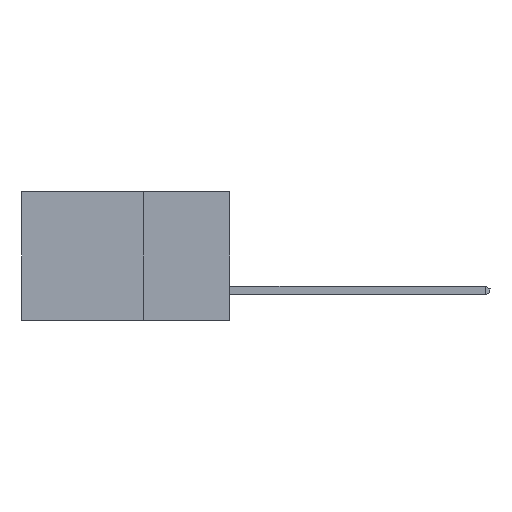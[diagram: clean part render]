
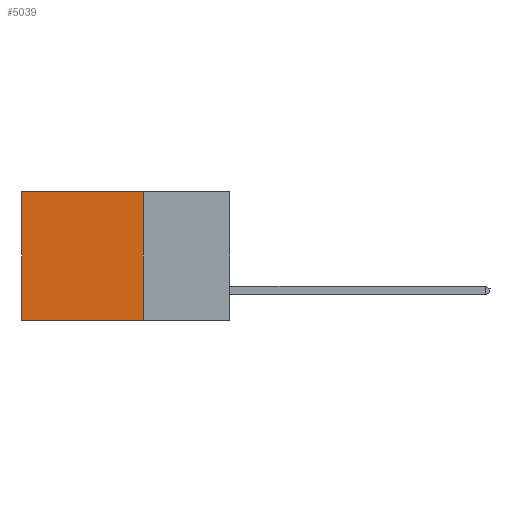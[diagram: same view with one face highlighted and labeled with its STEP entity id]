
A CAD part, left-side view. The second image highlights one B-rep face of the part: STEP entity #5039.
In plain terms, the highlighted planar face has unit normal (-1, 0, 0).
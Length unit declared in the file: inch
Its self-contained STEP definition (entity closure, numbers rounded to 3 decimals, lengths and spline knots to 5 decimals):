
#71 = AXIS2_PLACEMENT_3D ( 'NONE', #5232, #5134, #6572 ) ;
#992 = CARTESIAN_POINT ( 'NONE',  ( 0.298, 0.25, 0. ) ) ;
#1213 = CARTESIAN_POINT ( 'NONE',  ( 0.298, 0.6, -0.37 ) ) ;
#1658 = EDGE_CURVE ( 'NONE', #10944, #4196, #7610, .T. ) ;
#3226 = VECTOR ( 'NONE', #11026, 39.37008 ) ;
#4196 = VERTEX_POINT ( 'NONE', #11850 ) ;
#4516 = CARTESIAN_POINT ( 'NONE',  ( 0.298, 0.6, 0. ) ) ;
#4871 = DIRECTION ( 'NONE',  ( 0., 1., 0. ) ) ;
#5039 = ADVANCED_FACE ( 'NONE', ( #14715 ), #13053, .F. ) ;
#5134 = DIRECTION ( 'NONE',  ( 1., 0., 0. ) ) ;
#5232 = CARTESIAN_POINT ( 'NONE',  ( 0.298, 0.25, 0. ) ) ;
#6140 = EDGE_CURVE ( 'NONE', #4196, #11334, #9759, .T. ) ;
#6254 = EDGE_CURVE ( 'NONE', #7021, #11334, #13254, .T. ) ;
#6343 = DIRECTION ( 'NONE',  ( 0., 0., -1. ) ) ;
#6572 = DIRECTION ( 'NONE',  ( 0., 0., -1. ) ) ;
#7021 = VERTEX_POINT ( 'NONE', #11806 ) ;
#7163 = CARTESIAN_POINT ( 'NONE',  ( 0.298, 0.25, -0.37 ) ) ;
#7186 = VECTOR ( 'NONE', #4871, 39.37008 ) ;
#7610 = LINE ( 'NONE', #992, #15599 ) ;
#7684 = CARTESIAN_POINT ( 'NONE',  ( 0.298, 0.25, 0. ) ) ;
#8200 = LINE ( 'NONE', #16593, #7186 ) ;
#9149 = VECTOR ( 'NONE', #13655, 39.37008 ) ;
#9690 = EDGE_CURVE ( 'NONE', #10944, #7021, #8200, .T. ) ;
#9759 = LINE ( 'NONE', #7163, #3226 ) ;
#10654 = ORIENTED_EDGE ( 'NONE', *, *, #1658, .F. ) ;
#10944 = VERTEX_POINT ( 'NONE', #7684 ) ;
#11026 = DIRECTION ( 'NONE',  ( 0., 1., 0. ) ) ;
#11334 = VERTEX_POINT ( 'NONE', #1213 ) ;
#11806 = CARTESIAN_POINT ( 'NONE',  ( 0.298, 0.6, 0. ) ) ;
#11850 = CARTESIAN_POINT ( 'NONE',  ( 0.298, 0.25, -0.37 ) ) ;
#12497 = ORIENTED_EDGE ( 'NONE', *, *, #9690, .T. ) ;
#13053 = PLANE ( 'NONE',  #71 ) ;
#13254 = LINE ( 'NONE', #4516, #9149 ) ;
#13655 = DIRECTION ( 'NONE',  ( 0., 0., -1. ) ) ;
#13908 = ORIENTED_EDGE ( 'NONE', *, *, #6140, .F. ) ;
#14075 = ORIENTED_EDGE ( 'NONE', *, *, #6254, .T. ) ;
#14144 = EDGE_LOOP ( 'NONE', ( #14075, #13908, #10654, #12497 ) ) ;
#14715 = FACE_OUTER_BOUND ( 'NONE', #14144, .T. ) ;
#15599 = VECTOR ( 'NONE', #6343, 39.37008 ) ;
#16593 = CARTESIAN_POINT ( 'NONE',  ( 0.298, 0.25, 0. ) ) ;
